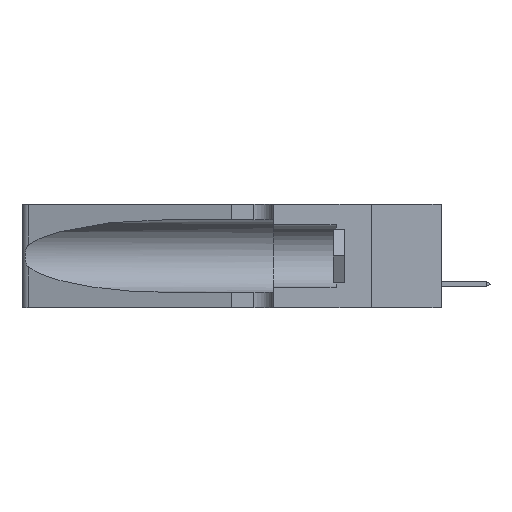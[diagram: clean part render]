
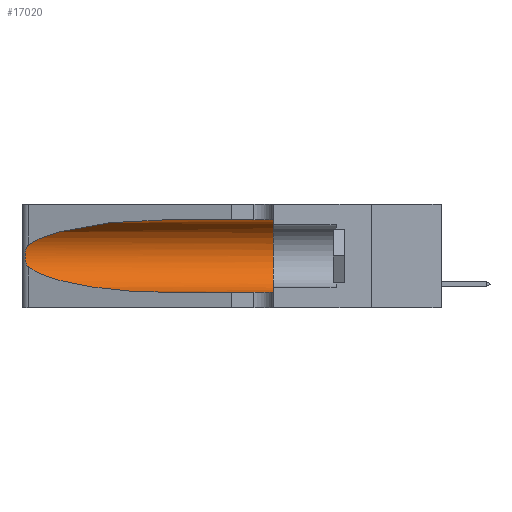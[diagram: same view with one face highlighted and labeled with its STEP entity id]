
A CAD part, left-side view. The second image highlights one B-rep face of the part: STEP entity #17020.
In plain terms, the highlighted cylindrical face has radius 3.308 mm (diameter 6.617 mm), a partial arc.
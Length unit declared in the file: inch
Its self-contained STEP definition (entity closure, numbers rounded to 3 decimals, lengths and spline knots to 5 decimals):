
#99 = CARTESIAN_POINT ( 'NONE',  ( 0.26075, 1.23896, 0.19203 ) ) ;
#214 = CARTESIAN_POINT ( 'NONE',  ( 0.25487, 1.22718, 0.22369 ) ) ;
#526 = DIRECTION ( 'NONE',  ( 0., 0., -1. ) ) ;
#922 = EDGE_CURVE ( 'NONE', #19011, #1113, #19594, .T. ) ;
#1113 = VERTEX_POINT ( 'NONE', #2491 ) ;
#1344 = DIRECTION ( 'NONE',  ( 0., -1., 0. ) ) ;
#1461 = CARTESIAN_POINT ( 'NONE',  ( 0.1305, 1.61858, 0.31525 ) ) ;
#1490 = CARTESIAN_POINT ( 'NONE',  ( 0.26017, 1.23833, 0.17102 ) ) ;
#1815 = CIRCLE ( 'NONE', #3664, 0.13025 ) ;
#2491 = CARTESIAN_POINT ( 'NONE',  ( 0.1305, 0.35, 0.05475 ) ) ;
#2593 = VERTEX_POINT ( 'NONE', #6178 ) ;
#3099 = CARTESIAN_POINT ( 'NONE',  ( 0.26075, 1.23896, 0.178 ) ) ;
#3547 = B_SPLINE_CURVE_WITH_KNOTS ( 'NONE', 3,
 ( #15205, #6054, #10551, #15145, #15322, #9209, #99, #3099, #1490, #6169, #12143, #10688, #18234, #13730 ),
 .UNSPECIFIED., .F., .F.,
 ( 4, 2, 2, 2, 2, 2, 4 ),
 ( 0., 0.00027, 0.00053, 0.00107, 0.0016, 0.00187, 0.00214 ),
 .UNSPECIFIED. ) ;
#3578 = DIRECTION ( 'NONE',  ( 0., -1., 0. ) ) ;
#3664 = AXIS2_PLACEMENT_3D ( 'NONE', #6022, #13307, #10244 ) ;
#3864 = EDGE_CURVE ( 'NONE', #2593, #19011, #16340, .T. ) ;
#4041 = EDGE_CURVE ( 'NONE', #9652, #15498, #10967, .T. ) ;
#4066 = CARTESIAN_POINT ( 'NONE',  ( 0.1305, 0.72297, 0.31525 ) ) ;
#4071 = CARTESIAN_POINT ( 'NONE',  ( 0.1305, 0.72297, 0.05475 ) ) ;
#6022 = CARTESIAN_POINT ( 'NONE',  ( 0.1305, 0.35, 0.185 ) ) ;
#6054 = CARTESIAN_POINT ( 'NONE',  ( 0.25555, 1.22994, 0.2215 ) ) ;
#6128 = ORIENTED_EDGE ( 'NONE', *, *, #18624, .F. ) ;
#6169 = CARTESIAN_POINT ( 'NONE',  ( 0.25856, 1.23593, 0.16098 ) ) ;
#6178 = CARTESIAN_POINT ( 'NONE',  ( 0.25487, 1.22718, 0.14631 ) ) ;
#6955 = ORIENTED_EDGE ( 'NONE', *, *, #16442, .T. ) ;
#7179 = ORIENTED_EDGE ( 'NONE', *, *, #3864, .T. ) ;
#7932 = AXIS2_PLACEMENT_3D ( 'NONE', #16914, #3578, #526 ) ;
#8184 = CARTESIAN_POINT ( 'NONE',  ( 0.1305, 0.35, 0.31525 ) ) ;
#8780 = CARTESIAN_POINT ( 'NONE',  ( 0.25487, 1.22718, 0.14631 ) ) ;
#9209 = CARTESIAN_POINT ( 'NONE',  ( 0.26018, 1.23835, 0.19895 ) ) ;
#9652 = VERTEX_POINT ( 'NONE', #18726 ) ;
#10244 = DIRECTION ( 'NONE',  ( 0., 0., 1. ) ) ;
#10365 = EDGE_LOOP ( 'NONE', ( #6955, #10484, #7179, #11938, #6128, #16809 ) ) ;
#10462 = FACE_OUTER_BOUND ( 'NONE', #10365, .T. ) ;
#10484 = ORIENTED_EDGE ( 'NONE', *, *, #12099, .T. ) ;
#10551 = CARTESIAN_POINT ( 'NONE',  ( 0.25639, 1.23184, 0.21858 ) ) ;
#10688 = CARTESIAN_POINT ( 'NONE',  ( 0.25639, 1.23186, 0.15144 ) ) ;
#10967 = LINE ( 'NONE', #1461, #15010 ) ;
#11541 = VECTOR ( 'NONE', #13166, 39.37008 ) ;
#11938 = ORIENTED_EDGE ( 'NONE', *, *, #922, .T. ) ;
#12099 = EDGE_CURVE ( 'NONE', #14357, #2593, #3547, .T. ) ;
#12143 = CARTESIAN_POINT ( 'NONE',  ( 0.25789, 1.23486, 0.15765 ) ) ;
#12798 = CARTESIAN_POINT ( 'NONE',  ( 0.1305, 0.72297, 0.05475 ) ) ;
#13166 = DIRECTION ( 'NONE',  ( 0., -1., 0. ) ) ;
#13196 = CARTESIAN_POINT ( 'NONE',  ( 0.18966, 0.96281, 0.05475 ) ) ;
#13307 = DIRECTION ( 'NONE',  ( 0., 1., 0. ) ) ;
#13452 = CARTESIAN_POINT ( 'NONE',  ( 0.25487, 1.22718, 0.22369 ) ) ;
#13730 = CARTESIAN_POINT ( 'NONE',  ( 0.25487, 1.22718, 0.14631 ) ) ;
#14357 = VERTEX_POINT ( 'NONE', #214 ) ;
#15010 = VECTOR ( 'NONE', #1344, 39.37008 ) ;
#15045 = CARTESIAN_POINT ( 'NONE',  ( 0.1305, 1.61858, 0.05475 ) ) ;
#15145 = CARTESIAN_POINT ( 'NONE',  ( 0.25787, 1.23484, 0.2124 ) ) ;
#15205 = CARTESIAN_POINT ( 'NONE',  ( 0.25487, 1.22718, 0.22369 ) ) ;
#15322 = CARTESIAN_POINT ( 'NONE',  ( 0.25854, 1.2359, 0.20912 ) ) ;
#15498 = VERTEX_POINT ( 'NONE', #8184 ) ;
#15853 =( BOUNDED_CURVE ( )  B_SPLINE_CURVE ( 3, ( #4066, #19286, #16490, #13452 ),
 .UNSPECIFIED., .F., .T. ) 
 B_SPLINE_CURVE_WITH_KNOTS ( ( 4, 4 ),
 ( 1.5708, 2.84003 ),
 .UNSPECIFIED. ) 
 CURVE ( )  GEOMETRIC_REPRESENTATION_ITEM ( )  RATIONAL_B_SPLINE_CURVE ( ( 1., 0.87, 0.87, 1. ) ) 
 REPRESENTATION_ITEM ( '' )  );
#16340 =( BOUNDED_CURVE ( )  B_SPLINE_CURVE ( 3, ( #8780, #18021, #13196, #4071 ),
 .UNSPECIFIED., .F., .F. ) 
 B_SPLINE_CURVE_WITH_KNOTS ( ( 4, 4 ),
 ( 3.44316, 4.71239 ),
 .UNSPECIFIED. ) 
 CURVE ( )  GEOMETRIC_REPRESENTATION_ITEM ( )  RATIONAL_B_SPLINE_CURVE ( ( 1., 0.87, 0.87, 1. ) ) 
 REPRESENTATION_ITEM ( '' )  );
#16442 = EDGE_CURVE ( 'NONE', #9652, #14357, #15853, .T. ) ;
#16490 = CARTESIAN_POINT ( 'NONE',  ( 0.2373, 1.15595, 0.28018 ) ) ;
#16809 = ORIENTED_EDGE ( 'NONE', *, *, #4041, .F. ) ;
#16862 = CYLINDRICAL_SURFACE ( 'NONE', #7932, 0.13025 ) ;
#16914 = CARTESIAN_POINT ( 'NONE',  ( 0.1305, 1.61858, 0.185 ) ) ;
#17020 = ADVANCED_FACE ( 'NONE', ( #10462 ), #16862, .F. ) ;
#18021 = CARTESIAN_POINT ( 'NONE',  ( 0.2373, 1.15595, 0.08982 ) ) ;
#18234 = CARTESIAN_POINT ( 'NONE',  ( 0.25555, 1.22993, 0.14849 ) ) ;
#18624 = EDGE_CURVE ( 'NONE', #15498, #1113, #1815, .T. ) ;
#18726 = CARTESIAN_POINT ( 'NONE',  ( 0.1305, 0.72297, 0.31525 ) ) ;
#19011 = VERTEX_POINT ( 'NONE', #12798 ) ;
#19286 = CARTESIAN_POINT ( 'NONE',  ( 0.18966, 0.96281, 0.31525 ) ) ;
#19594 = LINE ( 'NONE', #15045, #11541 ) ;
